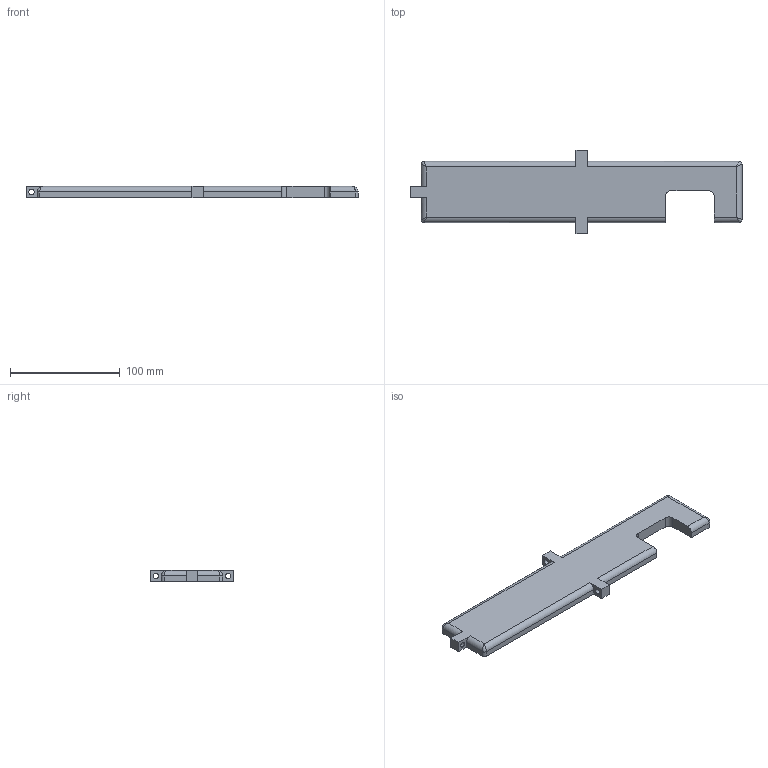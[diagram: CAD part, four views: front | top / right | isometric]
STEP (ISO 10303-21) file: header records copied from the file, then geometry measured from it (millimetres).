
FILE_DESCRIPTION (( 'STEP AP214' ), '1' );
FILE_NAME ('frame_top.STEP', '2013-09-24T00:00:19', ( '' ), ( '' ), 'SwSTEP 2.0', 'SolidWorks 2013', '' );
FILE_SCHEMA (( 'AUTOMOTIVE_DESIGN' ));
Length unit declared in the file: inch
Products named in the file (1): frame_top
Bounding box: 303.02 x 76.2 x 10.16 mm (x, y, z)
Volume: 152471.6 mm3; surface area: 38033.7 mm2
Topology: 1 solids, 1 shells, 46 faces, 124 edges, 76 vertices
Faces by surface type: plane 22, cylinder 20, bspline 4
Entity records: 1624 total; most frequent: CARTESIAN_POINT 455, ORIENTED_EDGE 240, DIRECTION 230, EDGE_CURVE 120, LINE 80, VECTOR 80, VERTEX_POINT 76, AXIS2_PLACEMENT_3D 75
